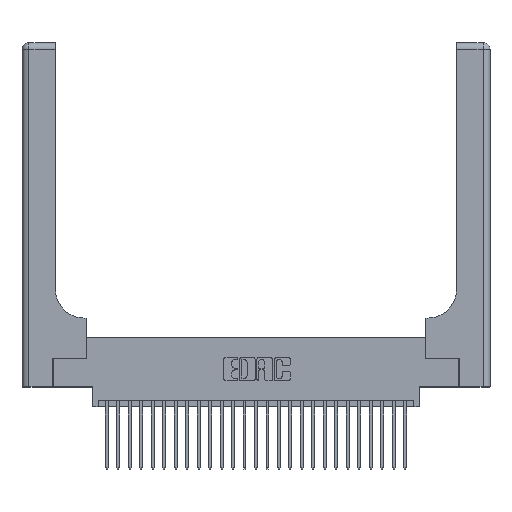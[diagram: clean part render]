
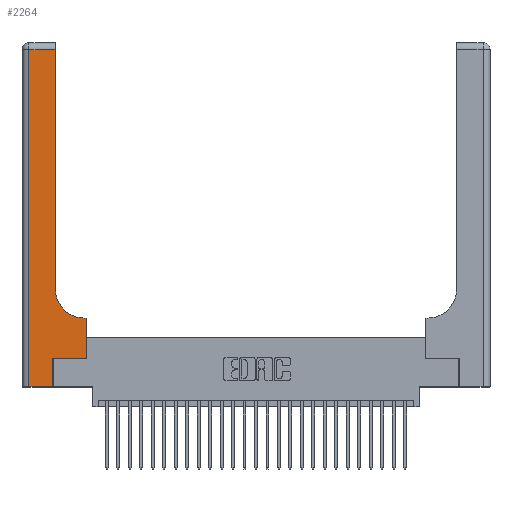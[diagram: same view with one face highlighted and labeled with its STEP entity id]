
A CAD part, top view. The second image highlights one B-rep face of the part: STEP entity #2264.
In plain terms, the highlighted planar face has unit normal (0, 0, 1).
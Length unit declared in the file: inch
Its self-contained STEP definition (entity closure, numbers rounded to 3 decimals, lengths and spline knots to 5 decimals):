
#281 = ORIENTED_EDGE ( 'NONE', *, *, #21240, .T. ) ;
#1257 = CARTESIAN_POINT ( 'NONE',  ( 0.06, 0., 0.37 ) ) ;
#1614 = AXIS2_PLACEMENT_3D ( 'NONE', #1863, #3879, #25977 ) ;
#1795 = CARTESIAN_POINT ( 'NONE',  ( 0.269, 0., 0.37 ) ) ;
#1863 = CARTESIAN_POINT ( 'NONE',  ( 0.5415, 0.85, 0.37 ) ) ;
#2264 = ADVANCED_FACE ( 'NONE', ( #15940 ), #15186, .F. ) ;
#2708 = ORIENTED_EDGE ( 'NONE', *, *, #19843, .T. ) ;
#2997 = VECTOR ( 'NONE', #24360, 39.37008 ) ;
#3748 = VECTOR ( 'NONE', #18974, 39.37008 ) ;
#3879 = DIRECTION ( 'NONE',  ( 0., 0., -1. ) ) ;
#4149 = DIRECTION ( 'NONE',  ( 0., 1., 0. ) ) ;
#4664 = CARTESIAN_POINT ( 'NONE',  ( 0.2915, 2.94, 0.37 ) ) ;
#5392 = DIRECTION ( 'NONE',  ( 0., 1., 0. ) ) ;
#5531 = LINE ( 'NONE', #12764, #14554 ) ;
#5745 = CARTESIAN_POINT ( 'NONE',  ( 0.06, 3., 0.37 ) ) ;
#6199 = VECTOR ( 'NONE', #24410, 39.37008 ) ;
#6401 = CARTESIAN_POINT ( 'NONE',  ( 0.5585, 0.25, 0.37 ) ) ;
#6482 = ORIENTED_EDGE ( 'NONE', *, *, #14718, .T. ) ;
#6565 = CARTESIAN_POINT ( 'NONE',  ( 0., 0., 0.37 ) ) ;
#6966 = VECTOR ( 'NONE', #26332, 39.37008 ) ;
#7049 = CARTESIAN_POINT ( 'NONE',  ( 0., 2.94, 0.37 ) ) ;
#7755 = ORIENTED_EDGE ( 'NONE', *, *, #18084, .T. ) ;
#8365 = LINE ( 'NONE', #6565, #6966 ) ;
#8571 = VERTEX_POINT ( 'NONE', #16023 ) ;
#8603 = VECTOR ( 'NONE', #12773, 39.37008 ) ;
#9096 = VERTEX_POINT ( 'NONE', #4664 ) ;
#10257 = LINE ( 'NONE', #6401, #2997 ) ;
#10610 = VERTEX_POINT ( 'NONE', #1257 ) ;
#10795 = EDGE_CURVE ( 'NONE', #8571, #23620, #16073, .T. ) ;
#12764 = CARTESIAN_POINT ( 'NONE',  ( 0.269, 0., 0.37 ) ) ;
#12773 = DIRECTION ( 'NONE',  ( 0., -1., 0. ) ) ;
#13157 = DIRECTION ( 'NONE',  ( -1., 0., 0. ) ) ;
#13456 = ORIENTED_EDGE ( 'NONE', *, *, #19991, .T. ) ;
#13926 = EDGE_CURVE ( 'NONE', #23497, #21600, #5531, .T. ) ;
#14554 = VECTOR ( 'NONE', #4149, 39.37008 ) ;
#14665 = VERTEX_POINT ( 'NONE', #18171 ) ;
#14718 = EDGE_CURVE ( 'NONE', #14665, #10610, #26168, .T. ) ;
#14841 = VECTOR ( 'NONE', #5392, 39.37008 ) ;
#15186 = PLANE ( 'NONE',  #25448 ) ;
#15679 = CARTESIAN_POINT ( 'NONE',  ( 0.2915, 0.6, 0.37 ) ) ;
#15940 = FACE_OUTER_BOUND ( 'NONE', #25010, .T. ) ;
#16023 = CARTESIAN_POINT ( 'NONE',  ( 0.5415, 0.6, 0.37 ) ) ;
#16073 = CIRCLE ( 'NONE', #1614, 0.25 ) ;
#18084 = EDGE_CURVE ( 'NONE', #9096, #14665, #20438, .T. ) ;
#18171 = CARTESIAN_POINT ( 'NONE',  ( 0.06, 2.94, 0.37 ) ) ;
#18974 = DIRECTION ( 'NONE',  ( 1., 0., 0. ) ) ;
#19843 = EDGE_CURVE ( 'NONE', #23445, #8571, #28244, .T. ) ;
#19991 = EDGE_CURVE ( 'NONE', #21600, #25840, #28211, .T. ) ;
#19994 = LINE ( 'NONE', #27362, #14841 ) ;
#20324 = EDGE_CURVE ( 'NONE', #23620, #9096, #19994, .T. ) ;
#20438 = LINE ( 'NONE', #7049, #24567 ) ;
#20443 = DIRECTION ( 'NONE',  ( -1., 0., 0. ) ) ;
#21240 = EDGE_CURVE ( 'NONE', #25840, #23445, #10257, .T. ) ;
#21568 = ORIENTED_EDGE ( 'NONE', *, *, #10795, .T. ) ;
#21600 = VERTEX_POINT ( 'NONE', #27496 ) ;
#22591 = CARTESIAN_POINT ( 'NONE',  ( 0.5585, 0.25, 0.37 ) ) ;
#23336 = CARTESIAN_POINT ( 'NONE',  ( 0.269, 0.25, 0.37 ) ) ;
#23378 = CARTESIAN_POINT ( 'NONE',  ( 0., 3., 0.37 ) ) ;
#23445 = VERTEX_POINT ( 'NONE', #23920 ) ;
#23497 = VERTEX_POINT ( 'NONE', #1795 ) ;
#23620 = VERTEX_POINT ( 'NONE', #24198 ) ;
#23726 = ORIENTED_EDGE ( 'NONE', *, *, #13926, .T. ) ;
#23920 = CARTESIAN_POINT ( 'NONE',  ( 0.5585, 0.6, 0.37 ) ) ;
#24198 = CARTESIAN_POINT ( 'NONE',  ( 0.2915, 0.85, 0.37 ) ) ;
#24360 = DIRECTION ( 'NONE',  ( 0., 1., 0. ) ) ;
#24410 = DIRECTION ( 'NONE',  ( -1., 0., 0. ) ) ;
#24567 = VECTOR ( 'NONE', #13157, 39.37008 ) ;
#25010 = EDGE_LOOP ( 'NONE', ( #27649, #7755, #6482, #27847, #23726, #13456, #281, #2708, #21568 ) ) ;
#25448 = AXIS2_PLACEMENT_3D ( 'NONE', #23378, #26498, #20443 ) ;
#25840 = VERTEX_POINT ( 'NONE', #22591 ) ;
#25977 = DIRECTION ( 'NONE',  ( 1., 0., 0. ) ) ;
#26168 = LINE ( 'NONE', #5745, #8603 ) ;
#26332 = DIRECTION ( 'NONE',  ( 1., 0., 0. ) ) ;
#26498 = DIRECTION ( 'NONE',  ( 0., 0., -1. ) ) ;
#26869 = EDGE_CURVE ( 'NONE', #10610, #23497, #8365, .T. ) ;
#27362 = CARTESIAN_POINT ( 'NONE',  ( 0.2915, 3., 0.37 ) ) ;
#27496 = CARTESIAN_POINT ( 'NONE',  ( 0.269, 0.25, 0.37 ) ) ;
#27649 = ORIENTED_EDGE ( 'NONE', *, *, #20324, .T. ) ;
#27847 = ORIENTED_EDGE ( 'NONE', *, *, #26869, .T. ) ;
#28211 = LINE ( 'NONE', #23336, #3748 ) ;
#28244 = LINE ( 'NONE', #15679, #6199 ) ;
